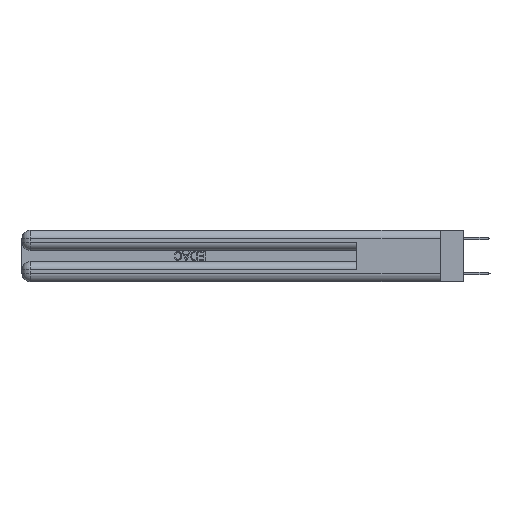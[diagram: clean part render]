
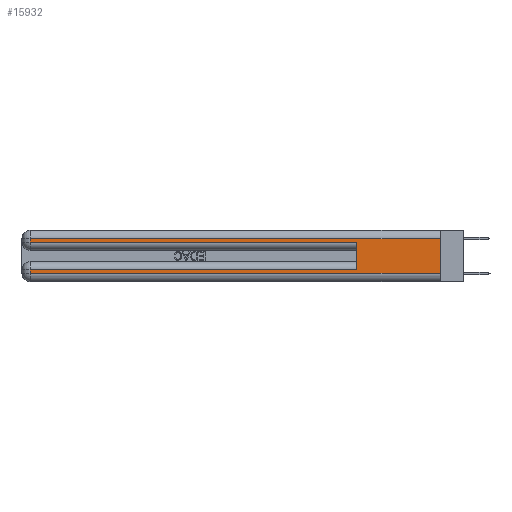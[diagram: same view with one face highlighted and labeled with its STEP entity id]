
A CAD part, left-side view. The second image highlights one B-rep face of the part: STEP entity #15932.
In plain terms, the highlighted planar face has unit normal (-1, 0, 0).
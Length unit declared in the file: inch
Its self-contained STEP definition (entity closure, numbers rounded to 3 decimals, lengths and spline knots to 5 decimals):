
#515 = DIRECTION ( 'NONE',  ( 1., 0., 0. ) ) ;
#1293 = VERTEX_POINT ( 'NONE', #5444 ) ;
#2509 = CARTESIAN_POINT ( 'NONE',  ( 0., 0.6, 0.145 ) ) ;
#2522 = VECTOR ( 'NONE', #19003, 39.37008 ) ;
#2659 = CARTESIAN_POINT ( 'NONE',  ( 0., 2.94, 0.31 ) ) ;
#3508 = VERTEX_POINT ( 'NONE', #29100 ) ;
#3596 = DIRECTION ( 'NONE',  ( 0., -1., 0. ) ) ;
#4465 = EDGE_CURVE ( 'NONE', #23026, #3508, #29805, .T. ) ;
#4598 = LINE ( 'NONE', #24374, #30463 ) ;
#5216 = CARTESIAN_POINT ( 'NONE',  ( 0., 0., 0.37 ) ) ;
#5444 = CARTESIAN_POINT ( 'NONE',  ( 0., 2.94, 0.085 ) ) ;
#6456 = CARTESIAN_POINT ( 'NONE',  ( 0., 2.94, 0.285 ) ) ;
#6627 = EDGE_CURVE ( 'NONE', #7234, #11846, #25460, .T. ) ;
#7007 = ORIENTED_EDGE ( 'NONE', *, *, #24940, .T. ) ;
#7012 = EDGE_CURVE ( 'NONE', #19364, #1293, #22535, .T. ) ;
#7234 = VERTEX_POINT ( 'NONE', #6456 ) ;
#7268 = CARTESIAN_POINT ( 'NONE',  ( 0., 0., 0.06 ) ) ;
#7948 = EDGE_CURVE ( 'NONE', #1293, #23881, #18143, .T. ) ;
#7965 = DIRECTION ( 'NONE',  ( 0., 0., 1. ) ) ;
#8033 = CARTESIAN_POINT ( 'NONE',  ( 0., 2.94, 0.37 ) ) ;
#8978 = CARTESIAN_POINT ( 'NONE',  ( 0., 0., 0.31 ) ) ;
#9732 = DIRECTION ( 'NONE',  ( 0., 1., 0. ) ) ;
#10319 = DIRECTION ( 'NONE',  ( 0., 0., -1. ) ) ;
#10489 = EDGE_CURVE ( 'NONE', #23881, #3508, #21883, .T. ) ;
#10594 = DIRECTION ( 'NONE',  ( 0., 0., -1. ) ) ;
#11642 = VECTOR ( 'NONE', #25137, 39.37008 ) ;
#11644 = VECTOR ( 'NONE', #25982, 39.37008 ) ;
#11743 = VERTEX_POINT ( 'NONE', #2659 ) ;
#11846 = VERTEX_POINT ( 'NONE', #13427 ) ;
#12435 = AXIS2_PLACEMENT_3D ( 'NONE', #22528, #515, #10319 ) ;
#12734 = PLANE ( 'NONE',  #12435 ) ;
#12893 = CARTESIAN_POINT ( 'NONE',  ( 0., 0., 0.085 ) ) ;
#13427 = CARTESIAN_POINT ( 'NONE',  ( 0., 0.6, 0.285 ) ) ;
#15166 = FACE_OUTER_BOUND ( 'NONE', #19143, .T. ) ;
#15932 = ADVANCED_FACE ( 'NONE', ( #15166 ), #12734, .F. ) ;
#18143 = LINE ( 'NONE', #30802, #11644 ) ;
#18413 = CARTESIAN_POINT ( 'NONE',  ( 0., 0., 0.285 ) ) ;
#18555 = ORIENTED_EDGE ( 'NONE', *, *, #7948, .T. ) ;
#19003 = DIRECTION ( 'NONE',  ( 0., -1., 0. ) ) ;
#19143 = EDGE_LOOP ( 'NONE', ( #31220, #7007, #23834, #22673, #22598, #26127, #18555, #19186 ) ) ;
#19186 = ORIENTED_EDGE ( 'NONE', *, *, #10489, .T. ) ;
#19364 = VERTEX_POINT ( 'NONE', #26416 ) ;
#20106 = VECTOR ( 'NONE', #10594, 39.37008 ) ;
#21402 = EDGE_CURVE ( 'NONE', #11743, #7234, #27630, .T. ) ;
#21797 = LINE ( 'NONE', #2509, #24821 ) ;
#21883 = LINE ( 'NONE', #7268, #2522 ) ;
#22528 = CARTESIAN_POINT ( 'NONE',  ( 0., 0., 0.37 ) ) ;
#22535 = LINE ( 'NONE', #12893, #27538 ) ;
#22598 = ORIENTED_EDGE ( 'NONE', *, *, #25035, .F. ) ;
#22673 = ORIENTED_EDGE ( 'NONE', *, *, #6627, .T. ) ;
#22694 = DIRECTION ( 'NONE',  ( 0., 1., 0. ) ) ;
#23026 = VERTEX_POINT ( 'NONE', #8978 ) ;
#23339 = CARTESIAN_POINT ( 'NONE',  ( 0., 2.94, 0.06 ) ) ;
#23834 = ORIENTED_EDGE ( 'NONE', *, *, #21402, .T. ) ;
#23881 = VERTEX_POINT ( 'NONE', #23339 ) ;
#24374 = CARTESIAN_POINT ( 'NONE',  ( 0., 0., 0.31 ) ) ;
#24821 = VECTOR ( 'NONE', #7965, 39.37008 ) ;
#24940 = EDGE_CURVE ( 'NONE', #23026, #11743, #4598, .T. ) ;
#25012 = VECTOR ( 'NONE', #3596, 39.37008 ) ;
#25035 = EDGE_CURVE ( 'NONE', #19364, #11846, #21797, .T. ) ;
#25137 = DIRECTION ( 'NONE',  ( 0., 0., -1. ) ) ;
#25460 = LINE ( 'NONE', #18413, #25012 ) ;
#25982 = DIRECTION ( 'NONE',  ( 0., 0., -1. ) ) ;
#26127 = ORIENTED_EDGE ( 'NONE', *, *, #7012, .T. ) ;
#26416 = CARTESIAN_POINT ( 'NONE',  ( 0., 0.6, 0.085 ) ) ;
#27538 = VECTOR ( 'NONE', #22694, 39.37008 ) ;
#27630 = LINE ( 'NONE', #8033, #20106 ) ;
#29100 = CARTESIAN_POINT ( 'NONE',  ( 0., 0., 0.06 ) ) ;
#29805 = LINE ( 'NONE', #5216, #11642 ) ;
#30463 = VECTOR ( 'NONE', #9732, 39.37008 ) ;
#30802 = CARTESIAN_POINT ( 'NONE',  ( 0., 2.94, 0.37 ) ) ;
#31220 = ORIENTED_EDGE ( 'NONE', *, *, #4465, .F. ) ;
